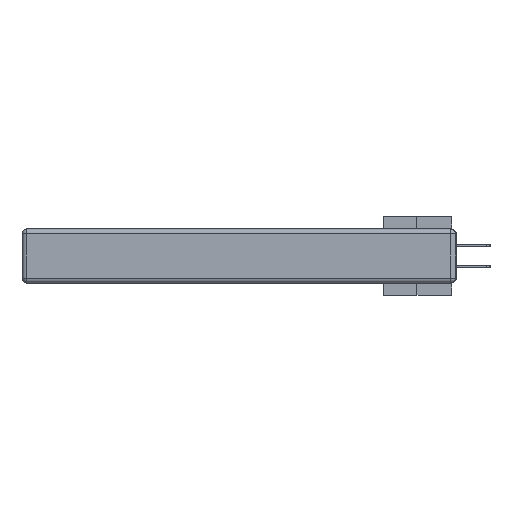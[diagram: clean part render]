
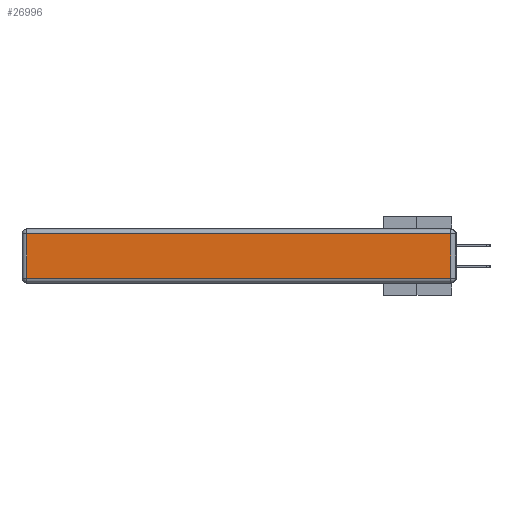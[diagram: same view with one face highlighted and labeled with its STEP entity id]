
A CAD part, left-side view. The second image highlights one B-rep face of the part: STEP entity #26996.
In plain terms, the highlighted planar face has unit normal (-1, 0, 0).
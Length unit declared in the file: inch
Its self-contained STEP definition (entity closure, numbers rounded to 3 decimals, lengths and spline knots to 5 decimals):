
#560 = VECTOR ( 'NONE', #3813, 39.37008 ) ;
#1022 = CARTESIAN_POINT ( 'NONE',  ( 0., 0.03, -0.313 ) ) ;
#1978 = ORIENTED_EDGE ( 'NONE', *, *, #30296, .T. ) ;
#2705 = VECTOR ( 'NONE', #21754, 39.37008 ) ;
#2815 = CARTESIAN_POINT ( 'NONE',  ( 0., 2.72, -0.343 ) ) ;
#3813 = DIRECTION ( 'NONE',  ( 0., 0., 1. ) ) ;
#5707 = AXIS2_PLACEMENT_3D ( 'NONE', #36772, #24377, #33337 ) ;
#10155 = CARTESIAN_POINT ( 'NONE',  ( 0., 0.03, -0.343 ) ) ;
#11157 = DIRECTION ( 'NONE',  ( 0., 1., 0. ) ) ;
#12815 = EDGE_CURVE ( 'NONE', #16860, #21068, #29251, .T. ) ;
#13374 = FACE_OUTER_BOUND ( 'NONE', #16483, .T. ) ;
#16483 = EDGE_LOOP ( 'NONE', ( #1978, #26372, #23870, #32882 ) ) ;
#16860 = VERTEX_POINT ( 'NONE', #32228 ) ;
#17439 = LINE ( 'NONE', #29693, #25049 ) ;
#17962 = EDGE_CURVE ( 'NONE', #35403, #16860, #17439, .T. ) ;
#21068 = VERTEX_POINT ( 'NONE', #35685 ) ;
#21543 = PLANE ( 'NONE',  #5707 ) ;
#21754 = DIRECTION ( 'NONE',  ( 0., -1., 0. ) ) ;
#23643 = LINE ( 'NONE', #27379, #2705 ) ;
#23870 = ORIENTED_EDGE ( 'NONE', *, *, #17962, .T. ) ;
#24377 = DIRECTION ( 'NONE',  ( -1., 0., 0. ) ) ;
#24610 = VERTEX_POINT ( 'NONE', #1022 ) ;
#25049 = VECTOR ( 'NONE', #11157, 39.37008 ) ;
#25334 = LINE ( 'NONE', #10155, #560 ) ;
#26372 = ORIENTED_EDGE ( 'NONE', *, *, #37491, .T. ) ;
#26889 = CARTESIAN_POINT ( 'NONE',  ( 0., 0.03, -0.03 ) ) ;
#26996 = ADVANCED_FACE ( 'NONE', ( #13374 ), #21543, .T. ) ;
#27379 = CARTESIAN_POINT ( 'NONE',  ( 0., 0., -0.313 ) ) ;
#29251 = LINE ( 'NONE', #2815, #32132 ) ;
#29693 = CARTESIAN_POINT ( 'NONE',  ( 0., 2.75, -0.03 ) ) ;
#30296 = EDGE_CURVE ( 'NONE', #21068, #24610, #23643, .T. ) ;
#32132 = VECTOR ( 'NONE', #36366, 39.37008 ) ;
#32228 = CARTESIAN_POINT ( 'NONE',  ( 0., 2.72, -0.03 ) ) ;
#32882 = ORIENTED_EDGE ( 'NONE', *, *, #12815, .T. ) ;
#33337 = DIRECTION ( 'NONE',  ( 0., 0., 1. ) ) ;
#35403 = VERTEX_POINT ( 'NONE', #26889 ) ;
#35685 = CARTESIAN_POINT ( 'NONE',  ( 0., 2.72, -0.313 ) ) ;
#36366 = DIRECTION ( 'NONE',  ( 0., 0., -1. ) ) ;
#36772 = CARTESIAN_POINT ( 'NONE',  ( 0., 0., -0.343 ) ) ;
#37491 = EDGE_CURVE ( 'NONE', #24610, #35403, #25334, .T. ) ;
